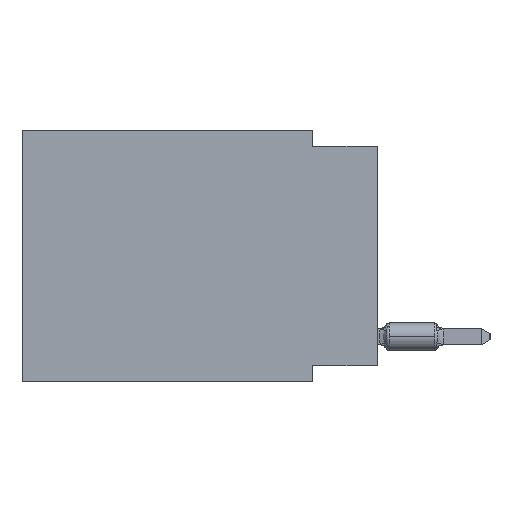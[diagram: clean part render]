
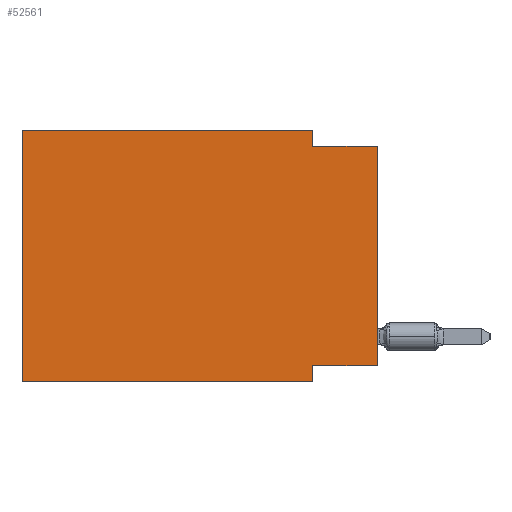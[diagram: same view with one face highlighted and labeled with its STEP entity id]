
A CAD part, left-side view. The second image highlights one B-rep face of the part: STEP entity #52561.
In plain terms, the highlighted planar face has unit normal (-1, 0, 0).
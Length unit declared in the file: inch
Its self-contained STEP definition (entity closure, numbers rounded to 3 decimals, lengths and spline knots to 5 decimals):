
#1395 = CARTESIAN_POINT ( 'NONE',  ( 0., 0., 0. ) ) ;
#2392 = DIRECTION ( 'NONE',  ( 0., -1., 0. ) ) ;
#3552 = CARTESIAN_POINT ( 'NONE',  ( 0., 0.1, 0. ) ) ;
#5344 = VERTEX_POINT ( 'NONE', #10001 ) ;
#5462 = ORIENTED_EDGE ( 'NONE', *, *, #11606, .F. ) ;
#5866 = VERTEX_POINT ( 'NONE', #24701 ) ;
#7019 = EDGE_CURVE ( 'NONE', #59681, #5344, #30489, .T. ) ;
#7248 = ORIENTED_EDGE ( 'NONE', *, *, #15523, .T. ) ;
#7494 = EDGE_LOOP ( 'NONE', ( #27421, #58569, #5462, #27253, #60911, #7248, #9907, #26537 ) ) ;
#7837 = LINE ( 'NONE', #37683, #62778 ) ;
#9332 = LINE ( 'NONE', #62017, #38051 ) ;
#9672 = DIRECTION ( 'NONE',  ( 0., 0., -1. ) ) ;
#9907 = ORIENTED_EDGE ( 'NONE', *, *, #7019, .F. ) ;
#10001 = CARTESIAN_POINT ( 'NONE',  ( 0., 0.1, -0.39 ) ) ;
#11606 = EDGE_CURVE ( 'NONE', #29452, #51637, #19618, .T. ) ;
#13252 = VECTOR ( 'NONE', #46266, 39.37008 ) ;
#14865 = CARTESIAN_POINT ( 'NONE',  ( 0., 0.55, 0. ) ) ;
#15118 = VERTEX_POINT ( 'NONE', #22239 ) ;
#15523 = EDGE_CURVE ( 'NONE', #15118, #5344, #26668, .T. ) ;
#17318 = EDGE_CURVE ( 'NONE', #62887, #59681, #9332, .T. ) ;
#19618 = LINE ( 'NONE', #53992, #58299 ) ;
#20249 = VECTOR ( 'NONE', #21921, 39.37008 ) ;
#21921 = DIRECTION ( 'NONE',  ( 0., 0., 1. ) ) ;
#22239 = CARTESIAN_POINT ( 'NONE',  ( 0., 0.55, -0.39 ) ) ;
#22840 = CARTESIAN_POINT ( 'NONE',  ( 0., 0.1, -0.025 ) ) ;
#23801 = DIRECTION ( 'NONE',  ( 0., 1., 0. ) ) ;
#23952 = CARTESIAN_POINT ( 'NONE',  ( 0., 0., -0.365 ) ) ;
#24701 = CARTESIAN_POINT ( 'NONE',  ( 0., 0., -0.025 ) ) ;
#25780 = DIRECTION ( 'NONE',  ( 1., 0., 0. ) ) ;
#26537 = ORIENTED_EDGE ( 'NONE', *, *, #17318, .F. ) ;
#26668 = LINE ( 'NONE', #60379, #13252 ) ;
#27253 = ORIENTED_EDGE ( 'NONE', *, *, #43845, .F. ) ;
#27421 = ORIENTED_EDGE ( 'NONE', *, *, #59233, .T. ) ;
#27928 = CARTESIAN_POINT ( 'NONE',  ( 0., 0., -0.025 ) ) ;
#28949 = EDGE_CURVE ( 'NONE', #15118, #30483, #43443, .T. ) ;
#29452 = VERTEX_POINT ( 'NONE', #3552 ) ;
#30483 = VERTEX_POINT ( 'NONE', #33418 ) ;
#30489 = LINE ( 'NONE', #55520, #37488 ) ;
#33418 = CARTESIAN_POINT ( 'NONE',  ( 0., 0.55, 0. ) ) ;
#34771 = DIRECTION ( 'NONE',  ( 0., 0., -1. ) ) ;
#37488 = VECTOR ( 'NONE', #55209, 39.37008 ) ;
#37554 = DIRECTION ( 'NONE',  ( 0., -1., 0. ) ) ;
#37683 = CARTESIAN_POINT ( 'NONE',  ( 0., 0.55, 0. ) ) ;
#38051 = VECTOR ( 'NONE', #23801, 39.37008 ) ;
#40208 = FACE_OUTER_BOUND ( 'NONE', #7494, .T. ) ;
#40232 = LINE ( 'NONE', #1395, #20249 ) ;
#42819 = CARTESIAN_POINT ( 'NONE',  ( 0., 0.55, 0. ) ) ;
#43443 = LINE ( 'NONE', #42819, #44416 ) ;
#43761 = DIRECTION ( 'NONE',  ( 0., 0., 1. ) ) ;
#43845 = EDGE_CURVE ( 'NONE', #30483, #29452, #7837, .T. ) ;
#44416 = VECTOR ( 'NONE', #43761, 39.37008 ) ;
#45781 = AXIS2_PLACEMENT_3D ( 'NONE', #14865, #25780, #34771 ) ;
#45835 = EDGE_CURVE ( 'NONE', #51637, #5866, #61643, .T. ) ;
#46266 = DIRECTION ( 'NONE',  ( 0., -1., 0. ) ) ;
#49824 = CARTESIAN_POINT ( 'NONE',  ( 0., 0.1, -0.365 ) ) ;
#49872 = PLANE ( 'NONE',  #45781 ) ;
#51637 = VERTEX_POINT ( 'NONE', #22840 ) ;
#52561 = ADVANCED_FACE ( 'NONE', ( #40208 ), #49872, .F. ) ;
#53992 = CARTESIAN_POINT ( 'NONE',  ( 0., 0.1, 0. ) ) ;
#55209 = DIRECTION ( 'NONE',  ( 0., 0., -1. ) ) ;
#55520 = CARTESIAN_POINT ( 'NONE',  ( 0., 0.1, -0.39 ) ) ;
#57824 = VECTOR ( 'NONE', #37554, 39.37008 ) ;
#58299 = VECTOR ( 'NONE', #9672, 39.37008 ) ;
#58569 = ORIENTED_EDGE ( 'NONE', *, *, #45835, .F. ) ;
#59233 = EDGE_CURVE ( 'NONE', #62887, #5866, #40232, .T. ) ;
#59681 = VERTEX_POINT ( 'NONE', #49824 ) ;
#60379 = CARTESIAN_POINT ( 'NONE',  ( 0., 0.55, -0.39 ) ) ;
#60911 = ORIENTED_EDGE ( 'NONE', *, *, #28949, .F. ) ;
#61643 = LINE ( 'NONE', #27928, #57824 ) ;
#62017 = CARTESIAN_POINT ( 'NONE',  ( 0., 0., -0.365 ) ) ;
#62778 = VECTOR ( 'NONE', #2392, 39.37008 ) ;
#62887 = VERTEX_POINT ( 'NONE', #23952 ) ;
